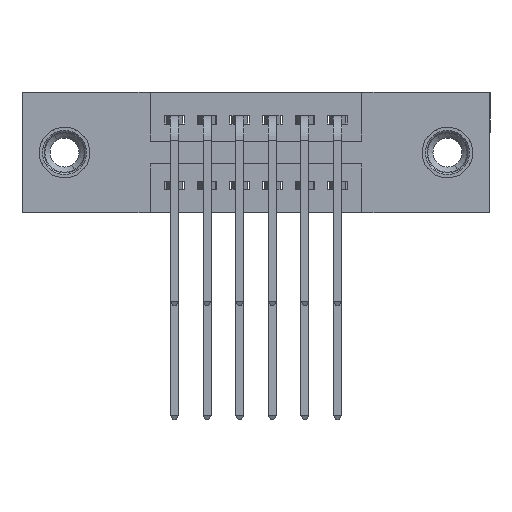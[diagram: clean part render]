
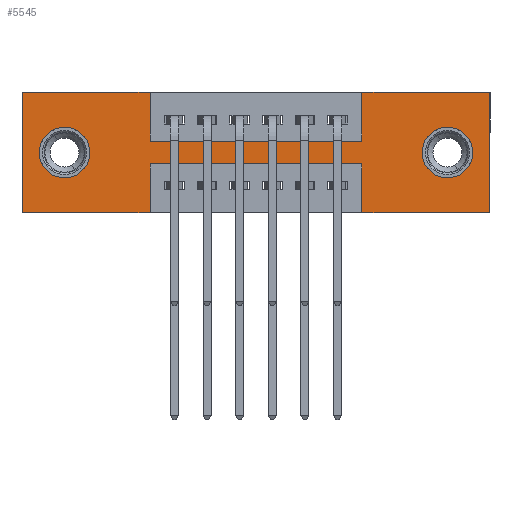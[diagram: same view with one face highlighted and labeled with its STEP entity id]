
A CAD part, front view. The second image highlights one B-rep face of the part: STEP entity #5545.
In plain terms, the highlighted planar face has unit normal (0, -1, 0).
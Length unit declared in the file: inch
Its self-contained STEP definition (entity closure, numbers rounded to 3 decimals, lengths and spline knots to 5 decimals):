
#23 = VECTOR ( 'NONE', #10344, 39.37008 ) ;
#144 = AXIS2_PLACEMENT_3D ( 'NONE', #12211, #5018, #13419 ) ;
#197 = EDGE_CURVE ( 'NONE', #1930, #12973, #9429, .T. ) ;
#313 = EDGE_LOOP ( 'NONE', ( #11557, #10867 ) ) ;
#338 = DIRECTION ( 'NONE',  ( 0., -1., 0. ) ) ;
#435 = FACE_BOUND ( 'NONE', #313, .T. ) ;
#554 = CIRCLE ( 'NONE', #7913, 0.078 ) ;
#729 = DIRECTION ( 'NONE',  ( 1., 0., 0. ) ) ;
#966 = LINE ( 'NONE', #14012, #10503 ) ;
#1070 = CARTESIAN_POINT ( 'NONE',  ( 1.435, 0., 0. ) ) ;
#1359 = DIRECTION ( 'NONE',  ( 0., 0., -1. ) ) ;
#1622 = CARTESIAN_POINT ( 'NONE',  ( 0., 0., -0.37 ) ) ;
#1780 = CARTESIAN_POINT ( 'NONE',  ( 1.0425, 0., 0. ) ) ;
#1806 = CARTESIAN_POINT ( 'NONE',  ( 0.3925, 0., -0.37 ) ) ;
#1930 = VERTEX_POINT ( 'NONE', #13358 ) ;
#2033 = EDGE_CURVE ( 'NONE', #5005, #9395, #3817, .T. ) ;
#2104 = DIRECTION ( 'NONE',  ( -1., 0., 0. ) ) ;
#2401 = LINE ( 'NONE', #9508, #15755 ) ;
#2621 = LINE ( 'NONE', #7320, #9231 ) ;
#2713 = ORIENTED_EDGE ( 'NONE', *, *, #197, .F. ) ;
#2736 = CARTESIAN_POINT ( 'NONE',  ( 1.0425, 0., 0. ) ) ;
#2924 = VECTOR ( 'NONE', #9554, 39.37008 ) ;
#3090 = CARTESIAN_POINT ( 'NONE',  ( 0., 0., 0. ) ) ;
#3106 = CARTESIAN_POINT ( 'NONE',  ( 1.305, 0., -0.185 ) ) ;
#3138 = VECTOR ( 'NONE', #15566, 39.37008 ) ;
#3298 = LINE ( 'NONE', #1806, #6281 ) ;
#3557 = DIRECTION ( 'NONE',  ( 0., 0., 1. ) ) ;
#3817 = LINE ( 'NONE', #1070, #13477 ) ;
#3951 = EDGE_CURVE ( 'NONE', #5877, #4832, #5349, .T. ) ;
#3955 = ORIENTED_EDGE ( 'NONE', *, *, #5550, .F. ) ;
#4313 = CARTESIAN_POINT ( 'NONE',  ( 0.3925, 0., 0. ) ) ;
#4420 = DIRECTION ( 'NONE',  ( 0., 0., -1. ) ) ;
#4433 = ORIENTED_EDGE ( 'NONE', *, *, #3951, .T. ) ;
#4502 = CARTESIAN_POINT ( 'NONE',  ( 0., 0., -0.37 ) ) ;
#4595 = ORIENTED_EDGE ( 'NONE', *, *, #13997, .F. ) ;
#4754 = VERTEX_POINT ( 'NONE', #5233 ) ;
#4781 = CARTESIAN_POINT ( 'NONE',  ( 1.435, 0., 0. ) ) ;
#4798 = VERTEX_POINT ( 'NONE', #11612 ) ;
#4832 = VERTEX_POINT ( 'NONE', #12865 ) ;
#5005 = VERTEX_POINT ( 'NONE', #4781 ) ;
#5018 = DIRECTION ( 'NONE',  ( 0., 1., 0. ) ) ;
#5103 = EDGE_CURVE ( 'NONE', #15915, #1930, #12833, .T. ) ;
#5233 = CARTESIAN_POINT ( 'NONE',  ( 0.3925, 0., -0.15 ) ) ;
#5335 = DIRECTION ( 'NONE',  ( 0., 1., 0. ) ) ;
#5349 = CIRCLE ( 'NONE', #9127, 0.078 ) ;
#5545 = ADVANCED_FACE ( 'NONE', ( #435, #7236, #10769 ), #7965, .T. ) ;
#5550 = EDGE_CURVE ( 'NONE', #11445, #4754, #13195, .T. ) ;
#5627 = CARTESIAN_POINT ( 'NONE',  ( 1.435, 0., -0.37 ) ) ;
#5636 = ORIENTED_EDGE ( 'NONE', *, *, #5927, .T. ) ;
#5864 = EDGE_LOOP ( 'NONE', ( #8896, #2713, #13140, #6097, #10719, #7783, #10216, #4595, #3955, #12866, #15774, #15316 ) ) ;
#5877 = VERTEX_POINT ( 'NONE', #12099 ) ;
#5927 = EDGE_CURVE ( 'NONE', #4832, #5877, #11871, .T. ) ;
#6053 = CARTESIAN_POINT ( 'NONE',  ( 1.0425, 0., -0.15 ) ) ;
#6097 = ORIENTED_EDGE ( 'NONE', *, *, #15683, .F. ) ;
#6116 = CARTESIAN_POINT ( 'NONE',  ( 0., 0., -0.37 ) ) ;
#6281 = VECTOR ( 'NONE', #12798, 39.37008 ) ;
#6298 = LINE ( 'NONE', #13083, #2924 ) ;
#6415 = CARTESIAN_POINT ( 'NONE',  ( 0., 0., -0.37 ) ) ;
#6435 = DIRECTION ( 'NONE',  ( 0., 1., 0. ) ) ;
#6581 = VECTOR ( 'NONE', #14525, 39.37008 ) ;
#6661 = DIRECTION ( 'NONE',  ( 0., 0., 1. ) ) ;
#6726 = LINE ( 'NONE', #6116, #12684 ) ;
#6803 = VECTOR ( 'NONE', #6661, 39.37008 ) ;
#7236 = FACE_BOUND ( 'NONE', #13115, .T. ) ;
#7320 = CARTESIAN_POINT ( 'NONE',  ( 0., 0., 0. ) ) ;
#7321 = DIRECTION ( 'NONE',  ( -1., 0., 0. ) ) ;
#7435 = VERTEX_POINT ( 'NONE', #13957 ) ;
#7711 = EDGE_CURVE ( 'NONE', #8909, #14634, #2621, .T. ) ;
#7783 = ORIENTED_EDGE ( 'NONE', *, *, #10945, .F. ) ;
#7821 = CARTESIAN_POINT ( 'NONE',  ( 1.0425, 0., -0.37 ) ) ;
#7894 = EDGE_CURVE ( 'NONE', #7435, #8909, #9765, .T. ) ;
#7913 = AXIS2_PLACEMENT_3D ( 'NONE', #3106, #11629, #4420 ) ;
#7963 = EDGE_CURVE ( 'NONE', #8294, #4798, #15015, .T. ) ;
#7965 = PLANE ( 'NONE',  #10793 ) ;
#8294 = VERTEX_POINT ( 'NONE', #11622 ) ;
#8450 = EDGE_CURVE ( 'NONE', #14634, #11445, #2401, .T. ) ;
#8896 = ORIENTED_EDGE ( 'NONE', *, *, #11433, .F. ) ;
#8909 = VERTEX_POINT ( 'NONE', #4502 ) ;
#9127 = AXIS2_PLACEMENT_3D ( 'NONE', #13588, #6435, #14821 ) ;
#9176 = DIRECTION ( 'NONE',  ( 0., 0., -1. ) ) ;
#9231 = VECTOR ( 'NONE', #3557, 39.37008 ) ;
#9395 = VERTEX_POINT ( 'NONE', #5627 ) ;
#9429 = LINE ( 'NONE', #14947, #13342 ) ;
#9508 = CARTESIAN_POINT ( 'NONE',  ( 0., 0., 0. ) ) ;
#9554 = DIRECTION ( 'NONE',  ( 1., 0., 0. ) ) ;
#9765 = LINE ( 'NONE', #6415, #6581 ) ;
#10216 = ORIENTED_EDGE ( 'NONE', *, *, #13261, .F. ) ;
#10344 = DIRECTION ( 'NONE',  ( 0., 0., -1. ) ) ;
#10503 = VECTOR ( 'NONE', #15184, 39.37008 ) ;
#10719 = ORIENTED_EDGE ( 'NONE', *, *, #2033, .F. ) ;
#10769 = FACE_OUTER_BOUND ( 'NONE', #5864, .T. ) ;
#10793 = AXIS2_PLACEMENT_3D ( 'NONE', #1622, #338, #9176 ) ;
#10867 = ORIENTED_EDGE ( 'NONE', *, *, #7963, .T. ) ;
#10945 = EDGE_CURVE ( 'NONE', #14024, #5005, #6298, .T. ) ;
#11433 = EDGE_CURVE ( 'NONE', #12973, #7435, #3298, .T. ) ;
#11445 = VERTEX_POINT ( 'NONE', #11651 ) ;
#11557 = ORIENTED_EDGE ( 'NONE', *, *, #14014, .T. ) ;
#11612 = CARTESIAN_POINT ( 'NONE',  ( 1.305, 0., -0.107 ) ) ;
#11622 = CARTESIAN_POINT ( 'NONE',  ( 1.305, 0., -0.263 ) ) ;
#11629 = DIRECTION ( 'NONE',  ( 0., 1., 0. ) ) ;
#11651 = CARTESIAN_POINT ( 'NONE',  ( 0.3925, 0., 0. ) ) ;
#11871 = CIRCLE ( 'NONE', #144, 0.078 ) ;
#12099 = CARTESIAN_POINT ( 'NONE',  ( 0.13, 0., -0.263 ) ) ;
#12211 = CARTESIAN_POINT ( 'NONE',  ( 0.13, 0., -0.185 ) ) ;
#12507 = CARTESIAN_POINT ( 'NONE',  ( 1.305, 0., -0.185 ) ) ;
#12684 = VECTOR ( 'NONE', #7321, 39.37008 ) ;
#12798 = DIRECTION ( 'NONE',  ( 0., 0., -1. ) ) ;
#12833 = LINE ( 'NONE', #14357, #3138 ) ;
#12865 = CARTESIAN_POINT ( 'NONE',  ( 0.13, 0., -0.107 ) ) ;
#12866 = ORIENTED_EDGE ( 'NONE', *, *, #8450, .F. ) ;
#12973 = VERTEX_POINT ( 'NONE', #15105 ) ;
#13083 = CARTESIAN_POINT ( 'NONE',  ( 0., 0., 0. ) ) ;
#13115 = EDGE_LOOP ( 'NONE', ( #5636, #4433 ) ) ;
#13139 = LINE ( 'NONE', #2736, #6803 ) ;
#13140 = ORIENTED_EDGE ( 'NONE', *, *, #5103, .F. ) ;
#13195 = LINE ( 'NONE', #4313, #23 ) ;
#13261 = EDGE_CURVE ( 'NONE', #14251, #14024, #13139, .T. ) ;
#13342 = VECTOR ( 'NONE', #2104, 39.37008 ) ;
#13358 = CARTESIAN_POINT ( 'NONE',  ( 1.0425, 0., -0.22 ) ) ;
#13419 = DIRECTION ( 'NONE',  ( 0., 0., 1. ) ) ;
#13477 = VECTOR ( 'NONE', #1359, 39.37008 ) ;
#13588 = CARTESIAN_POINT ( 'NONE',  ( 0.13, 0., -0.185 ) ) ;
#13728 = DIRECTION ( 'NONE',  ( 0., 0., -1. ) ) ;
#13957 = CARTESIAN_POINT ( 'NONE',  ( 0.3925, 0., -0.37 ) ) ;
#13997 = EDGE_CURVE ( 'NONE', #4754, #14251, #966, .T. ) ;
#14012 = CARTESIAN_POINT ( 'NONE',  ( 0.3925, 0., -0.15 ) ) ;
#14014 = EDGE_CURVE ( 'NONE', #4798, #8294, #554, .T. ) ;
#14024 = VERTEX_POINT ( 'NONE', #1780 ) ;
#14251 = VERTEX_POINT ( 'NONE', #6053 ) ;
#14357 = CARTESIAN_POINT ( 'NONE',  ( 1.0425, 0., -0.37 ) ) ;
#14525 = DIRECTION ( 'NONE',  ( -1., 0., 0. ) ) ;
#14634 = VERTEX_POINT ( 'NONE', #3090 ) ;
#14821 = DIRECTION ( 'NONE',  ( 0., 0., 1. ) ) ;
#14860 = AXIS2_PLACEMENT_3D ( 'NONE', #12507, #5335, #13728 ) ;
#14947 = CARTESIAN_POINT ( 'NONE',  ( 0.3925, 0., -0.22 ) ) ;
#15015 = CIRCLE ( 'NONE', #14860, 0.078 ) ;
#15105 = CARTESIAN_POINT ( 'NONE',  ( 0.3925, 0., -0.22 ) ) ;
#15184 = DIRECTION ( 'NONE',  ( 1., 0., 0. ) ) ;
#15316 = ORIENTED_EDGE ( 'NONE', *, *, #7894, .F. ) ;
#15566 = DIRECTION ( 'NONE',  ( 0., 0., 1. ) ) ;
#15683 = EDGE_CURVE ( 'NONE', #9395, #15915, #6726, .T. ) ;
#15755 = VECTOR ( 'NONE', #729, 39.37008 ) ;
#15774 = ORIENTED_EDGE ( 'NONE', *, *, #7711, .F. ) ;
#15915 = VERTEX_POINT ( 'NONE', #7821 ) ;
